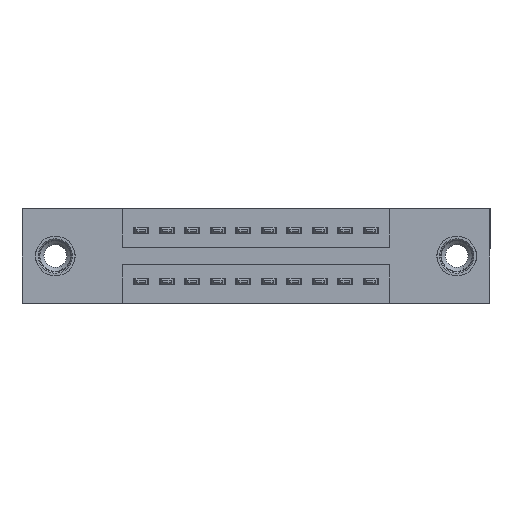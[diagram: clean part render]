
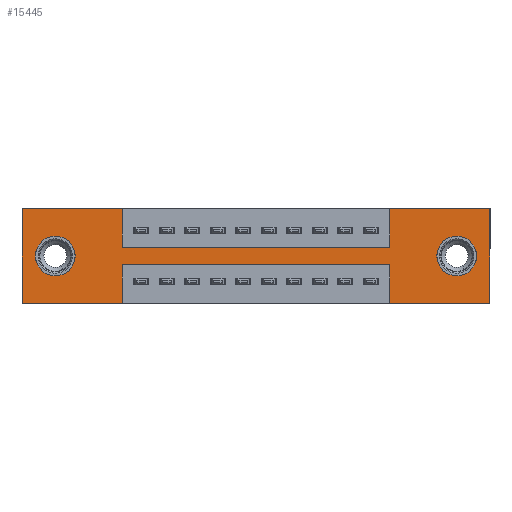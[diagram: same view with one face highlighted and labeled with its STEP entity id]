
A CAD part, front view. The second image highlights one B-rep face of the part: STEP entity #15445.
In plain terms, the highlighted planar face has unit normal (0, -1, 0).
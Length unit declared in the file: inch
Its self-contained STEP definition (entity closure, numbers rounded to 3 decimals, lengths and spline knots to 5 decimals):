
#486 = DIRECTION ( 'NONE',  ( 0., 0., -1. ) ) ;
#890 = CARTESIAN_POINT ( 'NONE',  ( 0.13, 0., -0.185 ) ) ;
#983 = VECTOR ( 'NONE', #3801, 39.37008 ) ;
#1024 = VERTEX_POINT ( 'NONE', #15726 ) ;
#1056 = EDGE_CURVE ( 'NONE', #3585, #1024, #11873, .T. ) ;
#1128 = ORIENTED_EDGE ( 'NONE', *, *, #14054, .F. ) ;
#1169 = DIRECTION ( 'NONE',  ( -1., 0., 0. ) ) ;
#1175 = DIRECTION ( 'NONE',  ( 0., 0., -1. ) ) ;
#1199 = VECTOR ( 'NONE', #12378, 39.37008 ) ;
#1281 = CARTESIAN_POINT ( 'NONE',  ( 1.705, 0., -0.107 ) ) ;
#1293 = LINE ( 'NONE', #8939, #8248 ) ;
#1329 = ORIENTED_EDGE ( 'NONE', *, *, #1056, .F. ) ;
#1683 = LINE ( 'NONE', #13367, #11625 ) ;
#1740 = VERTEX_POINT ( 'NONE', #11444 ) ;
#2111 = DIRECTION ( 'NONE',  ( 0., 1., 0. ) ) ;
#2182 = ORIENTED_EDGE ( 'NONE', *, *, #12259, .F. ) ;
#2251 = DIRECTION ( 'NONE',  ( 0., 0., 1. ) ) ;
#2262 = LINE ( 'NONE', #12654, #15502 ) ;
#2287 = AXIS2_PLACEMENT_3D ( 'NONE', #9879, #2111, #11164 ) ;
#2329 = CARTESIAN_POINT ( 'NONE',  ( 0.3925, 0., -0.15 ) ) ;
#2335 = EDGE_CURVE ( 'NONE', #8954, #2347, #1683, .T. ) ;
#2347 = VERTEX_POINT ( 'NONE', #10177 ) ;
#2398 = VERTEX_POINT ( 'NONE', #9127 ) ;
#2889 = VERTEX_POINT ( 'NONE', #13783 ) ;
#3237 = ORIENTED_EDGE ( 'NONE', *, *, #12828, .F. ) ;
#3355 = ORIENTED_EDGE ( 'NONE', *, *, #8660, .F. ) ;
#3585 = VERTEX_POINT ( 'NONE', #13922 ) ;
#3801 = DIRECTION ( 'NONE',  ( -1., 0., 0. ) ) ;
#4007 = DIRECTION ( 'NONE',  ( 0., 1., 0. ) ) ;
#4204 = VECTOR ( 'NONE', #5240, 39.37008 ) ;
#4223 = ORIENTED_EDGE ( 'NONE', *, *, #2335, .F. ) ;
#4369 = ORIENTED_EDGE ( 'NONE', *, *, #15198, .T. ) ;
#4428 = PLANE ( 'NONE',  #11362 ) ;
#4465 = LINE ( 'NONE', #15236, #13511 ) ;
#4482 = LINE ( 'NONE', #9001, #14313 ) ;
#4488 = DIRECTION ( 'NONE',  ( 0., 1., 0. ) ) ;
#4623 = FACE_BOUND ( 'NONE', #7469, .T. ) ;
#4673 = CARTESIAN_POINT ( 'NONE',  ( 0.3925, 0., 0. ) ) ;
#4736 = DIRECTION ( 'NONE',  ( 1., 0., 0. ) ) ;
#4824 = DIRECTION ( 'NONE',  ( 0., 0., 1. ) ) ;
#5003 = EDGE_CURVE ( 'NONE', #14028, #10454, #4482, .T. ) ;
#5240 = DIRECTION ( 'NONE',  ( 0., 0., -1. ) ) ;
#5369 = EDGE_CURVE ( 'NONE', #15608, #6988, #5678, .T. ) ;
#5404 = AXIS2_PLACEMENT_3D ( 'NONE', #11738, #4007, #13014 ) ;
#5490 = CARTESIAN_POINT ( 'NONE',  ( 1.4425, 0., -0.15 ) ) ;
#5516 = EDGE_CURVE ( 'NONE', #16017, #8276, #4465, .T. ) ;
#5571 = VERTEX_POINT ( 'NONE', #15513 ) ;
#5600 = VERTEX_POINT ( 'NONE', #7947 ) ;
#5678 = CIRCLE ( 'NONE', #2287, 0.078 ) ;
#5720 = CARTESIAN_POINT ( 'NONE',  ( 0., 0., -0.37 ) ) ;
#5742 = DIRECTION ( 'NONE',  ( 1., 0., 0. ) ) ;
#5848 = LINE ( 'NONE', #13718, #8908 ) ;
#5962 = CARTESIAN_POINT ( 'NONE',  ( 0.3925, 0., -0.37 ) ) ;
#6004 = CARTESIAN_POINT ( 'NONE',  ( 1.705, 0., -0.263 ) ) ;
#6943 = CIRCLE ( 'NONE', #5404, 0.078 ) ;
#6988 = VERTEX_POINT ( 'NONE', #1281 ) ;
#7000 = ORIENTED_EDGE ( 'NONE', *, *, #9598, .T. ) ;
#7469 = EDGE_LOOP ( 'NONE', ( #4369, #7000 ) ) ;
#7565 = LINE ( 'NONE', #8307, #13982 ) ;
#7947 = CARTESIAN_POINT ( 'NONE',  ( 0., 0., -0.37 ) ) ;
#8161 = EDGE_LOOP ( 'NONE', ( #13029, #16552 ) ) ;
#8248 = VECTOR ( 'NONE', #1169, 39.37008 ) ;
#8256 = AXIS2_PLACEMENT_3D ( 'NONE', #890, #10010, #2251 ) ;
#8276 = VERTEX_POINT ( 'NONE', #14618 ) ;
#8307 = CARTESIAN_POINT ( 'NONE',  ( 0., 0., 0. ) ) ;
#8340 = ORIENTED_EDGE ( 'NONE', *, *, #5516, .F. ) ;
#8347 = DIRECTION ( 'NONE',  ( 0., -1., 0. ) ) ;
#8526 = ORIENTED_EDGE ( 'NONE', *, *, #15680, .F. ) ;
#8660 = EDGE_CURVE ( 'NONE', #1024, #5571, #1293, .T. ) ;
#8908 = VECTOR ( 'NONE', #4736, 39.37008 ) ;
#8939 = CARTESIAN_POINT ( 'NONE',  ( 0., 0., -0.37 ) ) ;
#8954 = VERTEX_POINT ( 'NONE', #9600 ) ;
#9001 = CARTESIAN_POINT ( 'NONE',  ( 0.3925, 0., 0. ) ) ;
#9054 = EDGE_LOOP ( 'NONE', ( #2182, #4223, #3237, #3355, #1329, #1128, #8340, #8526, #12741, #12381, #11154, #12754 ) ) ;
#9127 = CARTESIAN_POINT ( 'NONE',  ( 0.13, 0., -0.263 ) ) ;
#9540 = VECTOR ( 'NONE', #4824, 39.37008 ) ;
#9598 = EDGE_CURVE ( 'NONE', #2398, #2889, #14204, .T. ) ;
#9600 = CARTESIAN_POINT ( 'NONE',  ( 1.4425, 0., -0.22 ) ) ;
#9879 = CARTESIAN_POINT ( 'NONE',  ( 1.705, 0., -0.185 ) ) ;
#9971 = CARTESIAN_POINT ( 'NONE',  ( 1.4425, 0., -0.37 ) ) ;
#10010 = DIRECTION ( 'NONE',  ( 0., 1., 0. ) ) ;
#10177 = CARTESIAN_POINT ( 'NONE',  ( 0.3925, 0., -0.22 ) ) ;
#10208 = CARTESIAN_POINT ( 'NONE',  ( 0., 0., -0.37 ) ) ;
#10336 = EDGE_CURVE ( 'NONE', #14182, #14028, #7565, .T. ) ;
#10454 = VERTEX_POINT ( 'NONE', #15027 ) ;
#10877 = LINE ( 'NONE', #2329, #11268 ) ;
#11154 = ORIENTED_EDGE ( 'NONE', *, *, #12434, .F. ) ;
#11164 = DIRECTION ( 'NONE',  ( 0., 0., -1. ) ) ;
#11268 = VECTOR ( 'NONE', #11351, 39.37008 ) ;
#11347 = LINE ( 'NONE', #10208, #983 ) ;
#11351 = DIRECTION ( 'NONE',  ( 1., 0., 0. ) ) ;
#11362 = AXIS2_PLACEMENT_3D ( 'NONE', #5720, #8347, #486 ) ;
#11378 = EDGE_CURVE ( 'NONE', #6988, #15608, #6943, .T. ) ;
#11444 = CARTESIAN_POINT ( 'NONE',  ( 0.3925, 0., -0.37 ) ) ;
#11471 = FACE_BOUND ( 'NONE', #8161, .T. ) ;
#11625 = VECTOR ( 'NONE', #13439, 39.37008 ) ;
#11738 = CARTESIAN_POINT ( 'NONE',  ( 1.705, 0., -0.185 ) ) ;
#11873 = LINE ( 'NONE', #14869, #4204 ) ;
#12200 = CARTESIAN_POINT ( 'NONE',  ( 0.13, 0., -0.185 ) ) ;
#12259 = EDGE_CURVE ( 'NONE', #2347, #1740, #15310, .T. ) ;
#12378 = DIRECTION ( 'NONE',  ( 0., 0., -1. ) ) ;
#12381 = ORIENTED_EDGE ( 'NONE', *, *, #10336, .F. ) ;
#12434 = EDGE_CURVE ( 'NONE', #5600, #14182, #2262, .T. ) ;
#12488 = EDGE_CURVE ( 'NONE', #1740, #5600, #11347, .T. ) ;
#12654 = CARTESIAN_POINT ( 'NONE',  ( 0., 0., 0. ) ) ;
#12741 = ORIENTED_EDGE ( 'NONE', *, *, #5003, .F. ) ;
#12754 = ORIENTED_EDGE ( 'NONE', *, *, #12488, .F. ) ;
#12828 = EDGE_CURVE ( 'NONE', #5571, #8954, #16277, .T. ) ;
#13014 = DIRECTION ( 'NONE',  ( 0., 0., -1. ) ) ;
#13029 = ORIENTED_EDGE ( 'NONE', *, *, #11378, .T. ) ;
#13351 = AXIS2_PLACEMENT_3D ( 'NONE', #12200, #4488, #13480 ) ;
#13367 = CARTESIAN_POINT ( 'NONE',  ( 0.3925, 0., -0.22 ) ) ;
#13439 = DIRECTION ( 'NONE',  ( -1., 0., 0. ) ) ;
#13480 = DIRECTION ( 'NONE',  ( 0., 0., 1. ) ) ;
#13511 = VECTOR ( 'NONE', #15294, 39.37008 ) ;
#13718 = CARTESIAN_POINT ( 'NONE',  ( 0., 0., 0. ) ) ;
#13783 = CARTESIAN_POINT ( 'NONE',  ( 0.13, 0., -0.107 ) ) ;
#13922 = CARTESIAN_POINT ( 'NONE',  ( 1.835, 0., 0. ) ) ;
#13926 = DIRECTION ( 'NONE',  ( 0., 0., 1. ) ) ;
#13982 = VECTOR ( 'NONE', #5742, 39.37008 ) ;
#14028 = VERTEX_POINT ( 'NONE', #4673 ) ;
#14037 = CARTESIAN_POINT ( 'NONE',  ( 0., 0., 0. ) ) ;
#14054 = EDGE_CURVE ( 'NONE', #8276, #3585, #5848, .T. ) ;
#14182 = VERTEX_POINT ( 'NONE', #14037 ) ;
#14204 = CIRCLE ( 'NONE', #13351, 0.078 ) ;
#14313 = VECTOR ( 'NONE', #1175, 39.37008 ) ;
#14618 = CARTESIAN_POINT ( 'NONE',  ( 1.4425, 0., 0. ) ) ;
#14869 = CARTESIAN_POINT ( 'NONE',  ( 1.835, 0., 0. ) ) ;
#15027 = CARTESIAN_POINT ( 'NONE',  ( 0.3925, 0., -0.15 ) ) ;
#15198 = EDGE_CURVE ( 'NONE', #2889, #2398, #15433, .T. ) ;
#15236 = CARTESIAN_POINT ( 'NONE',  ( 1.4425, 0., 0. ) ) ;
#15294 = DIRECTION ( 'NONE',  ( 0., 0., 1. ) ) ;
#15310 = LINE ( 'NONE', #5962, #1199 ) ;
#15433 = CIRCLE ( 'NONE', #8256, 0.078 ) ;
#15445 = ADVANCED_FACE ( 'NONE', ( #11471, #4623, #15625 ), #4428, .T. ) ;
#15502 = VECTOR ( 'NONE', #13926, 39.37008 ) ;
#15513 = CARTESIAN_POINT ( 'NONE',  ( 1.4425, 0., -0.37 ) ) ;
#15608 = VERTEX_POINT ( 'NONE', #6004 ) ;
#15625 = FACE_OUTER_BOUND ( 'NONE', #9054, .T. ) ;
#15680 = EDGE_CURVE ( 'NONE', #10454, #16017, #10877, .T. ) ;
#15726 = CARTESIAN_POINT ( 'NONE',  ( 1.835, 0., -0.37 ) ) ;
#16017 = VERTEX_POINT ( 'NONE', #5490 ) ;
#16277 = LINE ( 'NONE', #9971, #9540 ) ;
#16552 = ORIENTED_EDGE ( 'NONE', *, *, #5369, .T. ) ;
